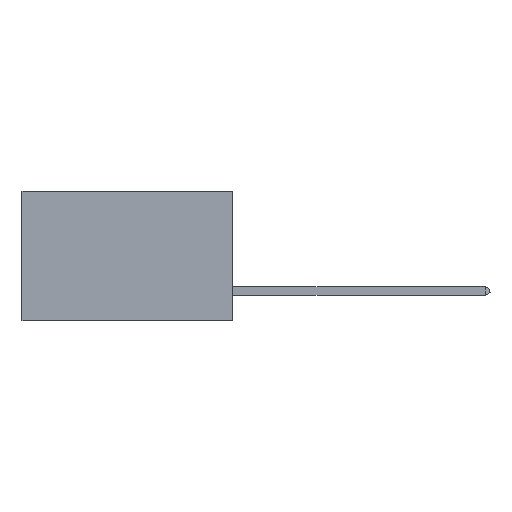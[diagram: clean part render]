
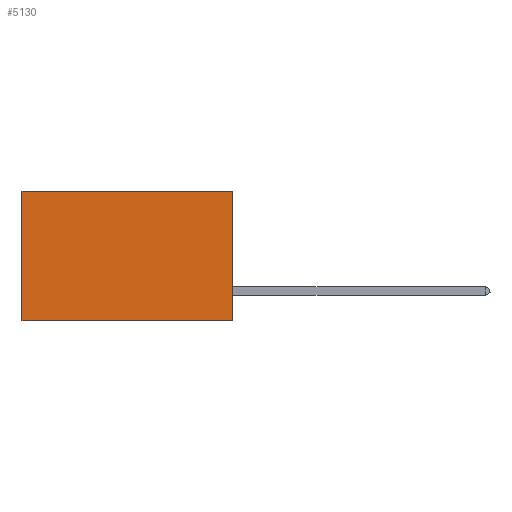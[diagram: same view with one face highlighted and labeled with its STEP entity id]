
A CAD part, left-side view. The second image highlights one B-rep face of the part: STEP entity #5130.
In plain terms, the highlighted planar face has unit normal (-1, 0, 0).
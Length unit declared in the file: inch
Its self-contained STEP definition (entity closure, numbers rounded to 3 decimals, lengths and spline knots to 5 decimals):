
#68 = VECTOR ( 'NONE', #133, 39.37008 ) ;
#133 = DIRECTION ( 'NONE',  ( 0., 0., -1. ) ) ;
#551 = CARTESIAN_POINT ( 'NONE',  ( 0.2875, 0., 0. ) ) ;
#2152 = DIRECTION ( 'NONE',  ( 0., 0., -1. ) ) ;
#3806 = ORIENTED_EDGE ( 'NONE', *, *, #30814, .F. ) ;
#4776 = VERTEX_POINT ( 'NONE', #551 ) ;
#5130 = ADVANCED_FACE ( 'NONE', ( #25791 ), #16145, .F. ) ;
#5199 = CARTESIAN_POINT ( 'NONE',  ( 0.2875, 0., 0. ) ) ;
#6620 = AXIS2_PLACEMENT_3D ( 'NONE', #5199, #22996, #2152 ) ;
#9016 = DIRECTION ( 'NONE',  ( 0., 0., -1. ) ) ;
#10865 = CARTESIAN_POINT ( 'NONE',  ( 0.2875, 0.6, 0. ) ) ;
#12344 = VECTOR ( 'NONE', #9016, 39.37008 ) ;
#14912 = ORIENTED_EDGE ( 'NONE', *, *, #35072, .T. ) ;
#16145 = PLANE ( 'NONE',  #6620 ) ;
#18232 = CARTESIAN_POINT ( 'NONE',  ( 0.2875, 0.6, -0.37 ) ) ;
#18482 = VERTEX_POINT ( 'NONE', #37845 ) ;
#18548 = LINE ( 'NONE', #10865, #68 ) ;
#19233 = ORIENTED_EDGE ( 'NONE', *, *, #29851, .F. ) ;
#21940 = CARTESIAN_POINT ( 'NONE',  ( 0.2875, 0., 0. ) ) ;
#22252 = EDGE_CURVE ( 'NONE', #18482, #37899, #18548, .T. ) ;
#22996 = DIRECTION ( 'NONE',  ( 1., 0., 0. ) ) ;
#24990 = LINE ( 'NONE', #44451, #35831 ) ;
#25791 = FACE_OUTER_BOUND ( 'NONE', #29201, .T. ) ;
#28377 = VECTOR ( 'NONE', #35892, 39.37008 ) ;
#29201 = EDGE_LOOP ( 'NONE', ( #29826, #19233, #3806, #14912 ) ) ;
#29826 = ORIENTED_EDGE ( 'NONE', *, *, #22252, .T. ) ;
#29851 = EDGE_CURVE ( 'NONE', #36759, #37899, #24990, .T. ) ;
#30814 = EDGE_CURVE ( 'NONE', #4776, #36759, #34631, .T. ) ;
#34631 = LINE ( 'NONE', #43614, #12344 ) ;
#35072 = EDGE_CURVE ( 'NONE', #4776, #18482, #39776, .T. ) ;
#35831 = VECTOR ( 'NONE', #37070, 39.37008 ) ;
#35892 = DIRECTION ( 'NONE',  ( 0., 1., 0. ) ) ;
#36356 = CARTESIAN_POINT ( 'NONE',  ( 0.2875, 0., -0.37 ) ) ;
#36759 = VERTEX_POINT ( 'NONE', #36356 ) ;
#37070 = DIRECTION ( 'NONE',  ( 0., 1., 0. ) ) ;
#37845 = CARTESIAN_POINT ( 'NONE',  ( 0.2875, 0.6, 0. ) ) ;
#37899 = VERTEX_POINT ( 'NONE', #18232 ) ;
#39776 = LINE ( 'NONE', #21940, #28377 ) ;
#43614 = CARTESIAN_POINT ( 'NONE',  ( 0.2875, 0., 0. ) ) ;
#44451 = CARTESIAN_POINT ( 'NONE',  ( 0.2875, 0., -0.37 ) ) ;
